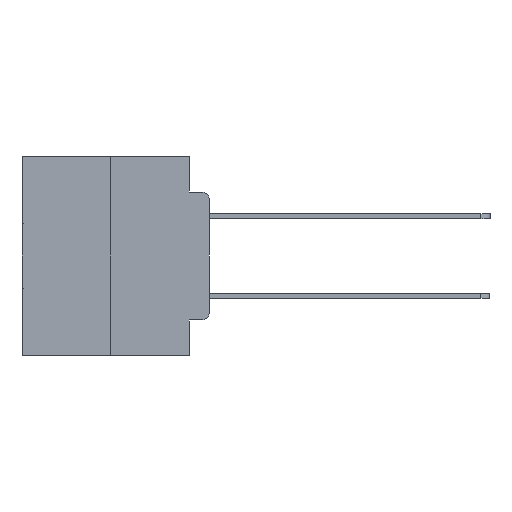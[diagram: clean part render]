
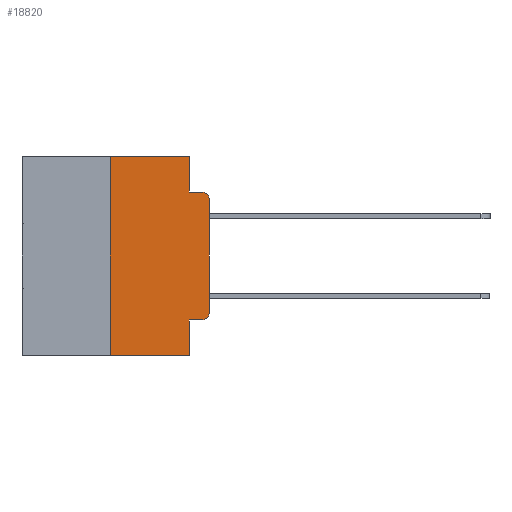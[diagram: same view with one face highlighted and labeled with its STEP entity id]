
A CAD part, left-side view. The second image highlights one B-rep face of the part: STEP entity #18820.
In plain terms, the highlighted planar face has unit normal (-1, 0, 0).
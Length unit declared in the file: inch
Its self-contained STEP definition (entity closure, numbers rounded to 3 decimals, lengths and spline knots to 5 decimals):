
#293 = DIRECTION ( 'NONE',  ( 0., 0., -1. ) ) ;
#661 = CARTESIAN_POINT ( 'NONE',  ( 0., 0., -0.1085 ) ) ;
#760 = VERTEX_POINT ( 'NONE', #27872 ) ;
#776 = ORIENTED_EDGE ( 'NONE', *, *, #23152, .F. ) ;
#808 = ORIENTED_EDGE ( 'NONE', *, *, #11839, .T. ) ;
#1389 = LINE ( 'NONE', #4992, #23170 ) ;
#1427 = CARTESIAN_POINT ( 'NONE',  ( 0., 0.473, 0. ) ) ;
#1507 = DIRECTION ( 'NONE',  ( 0., -1., 0. ) ) ;
#1617 = VERTEX_POINT ( 'NONE', #24075 ) ;
#1977 = LINE ( 'NONE', #11711, #16185 ) ;
#2202 = ORIENTED_EDGE ( 'NONE', *, *, #17604, .T. ) ;
#2776 = CARTESIAN_POINT ( 'NONE',  ( 0., 0.02, -0.3915 ) ) ;
#2945 = LINE ( 'NONE', #1427, #21610 ) ;
#3158 = VECTOR ( 'NONE', #23903, 39.37008 ) ;
#3261 = EDGE_CURVE ( 'NONE', #8089, #20990, #1389, .T. ) ;
#3321 = EDGE_CURVE ( 'NONE', #14280, #760, #9244, .T. ) ;
#3404 = VECTOR ( 'NONE', #19636, 39.37008 ) ;
#4658 = VECTOR ( 'NONE', #1507, 39.37008 ) ;
#4992 = CARTESIAN_POINT ( 'NONE',  ( 0., 0.25, 0. ) ) ;
#5052 = DIRECTION ( 'NONE',  ( 0., 0., -1. ) ) ;
#5710 = CARTESIAN_POINT ( 'NONE',  ( 0., 0.473, -0.5 ) ) ;
#6190 = VECTOR ( 'NONE', #25550, 39.37008 ) ;
#7208 = VERTEX_POINT ( 'NONE', #21252 ) ;
#7575 = DIRECTION ( 'NONE',  ( -1., 0., 0. ) ) ;
#7613 = VERTEX_POINT ( 'NONE', #661 ) ;
#7803 = DIRECTION ( 'NONE',  ( 0., 0., -1. ) ) ;
#8089 = VERTEX_POINT ( 'NONE', #12100 ) ;
#8682 = ORIENTED_EDGE ( 'NONE', *, *, #21087, .T. ) ;
#8787 = LINE ( 'NONE', #15295, #3404 ) ;
#9031 = ORIENTED_EDGE ( 'NONE', *, *, #3261, .F. ) ;
#9244 = LINE ( 'NONE', #18256, #3158 ) ;
#9692 = VERTEX_POINT ( 'NONE', #16600 ) ;
#10393 = EDGE_CURVE ( 'NONE', #7613, #760, #13295, .T. ) ;
#10438 = FACE_OUTER_BOUND ( 'NONE', #16031, .T. ) ;
#10463 = ORIENTED_EDGE ( 'NONE', *, *, #16174, .F. ) ;
#10605 = CARTESIAN_POINT ( 'NONE',  ( 0., 0.051, -0.5 ) ) ;
#10777 = LINE ( 'NONE', #12896, #4658 ) ;
#11406 = VECTOR ( 'NONE', #27967, 39.37008 ) ;
#11506 = ORIENTED_EDGE ( 'NONE', *, *, #3321, .F. ) ;
#11711 = CARTESIAN_POINT ( 'NONE',  ( 0., 0.051, 0. ) ) ;
#11839 = EDGE_CURVE ( 'NONE', #7208, #9692, #24347, .T. ) ;
#12100 = CARTESIAN_POINT ( 'NONE',  ( 0., 0.25, -0.5 ) ) ;
#12297 = LINE ( 'NONE', #18966, #6190 ) ;
#12302 = PLANE ( 'NONE',  #25947 ) ;
#12896 = CARTESIAN_POINT ( 'NONE',  ( 0., 0.051, -0.4115 ) ) ;
#13295 = CIRCLE ( 'NONE', #26937, 0.02 ) ;
#14280 = VERTEX_POINT ( 'NONE', #16419 ) ;
#15295 = CARTESIAN_POINT ( 'NONE',  ( 0., 0.051, 0. ) ) ;
#16031 = EDGE_LOOP ( 'NONE', ( #2202, #25005, #11506, #776, #26426, #9031, #8682, #10463, #18866, #808 ) ) ;
#16174 = EDGE_CURVE ( 'NONE', #1617, #16543, #1977, .T. ) ;
#16185 = VECTOR ( 'NONE', #293, 39.37008 ) ;
#16419 = CARTESIAN_POINT ( 'NONE',  ( 0., 0.051, -0.0885 ) ) ;
#16543 = VERTEX_POINT ( 'NONE', #10605 ) ;
#16600 = CARTESIAN_POINT ( 'NONE',  ( 0., 0., -0.3915 ) ) ;
#17285 = DIRECTION ( 'NONE',  ( 0., -1., 0. ) ) ;
#17604 = EDGE_CURVE ( 'NONE', #9692, #7613, #12297, .T. ) ;
#18256 = CARTESIAN_POINT ( 'NONE',  ( 0., 0.051, -0.0885 ) ) ;
#18400 = EDGE_CURVE ( 'NONE', #20990, #22371, #2945, .T. ) ;
#18599 = DIRECTION ( 'NONE',  ( -1., 0., 0. ) ) ;
#18820 = ADVANCED_FACE ( 'NONE', ( #10438 ), #12302, .F. ) ;
#18866 = ORIENTED_EDGE ( 'NONE', *, *, #19003, .T. ) ;
#18966 = CARTESIAN_POINT ( 'NONE',  ( 0., 0., 0. ) ) ;
#18998 = CARTESIAN_POINT ( 'NONE',  ( 0., 0.473, 0. ) ) ;
#19003 = EDGE_CURVE ( 'NONE', #1617, #7208, #10777, .T. ) ;
#19636 = DIRECTION ( 'NONE',  ( 0., 0., -1. ) ) ;
#19972 = AXIS2_PLACEMENT_3D ( 'NONE', #2776, #18599, #5052 ) ;
#20976 = CARTESIAN_POINT ( 'NONE',  ( 0., 0.25, 0. ) ) ;
#20990 = VERTEX_POINT ( 'NONE', #20976 ) ;
#21007 = CARTESIAN_POINT ( 'NONE',  ( 0., 0.02, -0.1085 ) ) ;
#21087 = EDGE_CURVE ( 'NONE', #8089, #16543, #27100, .T. ) ;
#21219 = DIRECTION ( 'NONE',  ( 1., 0., 0. ) ) ;
#21252 = CARTESIAN_POINT ( 'NONE',  ( 0., 0.02, -0.4115 ) ) ;
#21610 = VECTOR ( 'NONE', #17285, 39.37008 ) ;
#21815 = DIRECTION ( 'NONE',  ( 0., 0., 1. ) ) ;
#21941 = CARTESIAN_POINT ( 'NONE',  ( 0., 0.051, 0. ) ) ;
#22371 = VERTEX_POINT ( 'NONE', #21941 ) ;
#23152 = EDGE_CURVE ( 'NONE', #22371, #14280, #8787, .T. ) ;
#23170 = VECTOR ( 'NONE', #21815, 39.37008 ) ;
#23183 = DIRECTION ( 'NONE',  ( 0., 0., -1. ) ) ;
#23903 = DIRECTION ( 'NONE',  ( 0., -1., 0. ) ) ;
#24075 = CARTESIAN_POINT ( 'NONE',  ( 0., 0.051, -0.4115 ) ) ;
#24347 = CIRCLE ( 'NONE', #19972, 0.02 ) ;
#25005 = ORIENTED_EDGE ( 'NONE', *, *, #10393, .T. ) ;
#25550 = DIRECTION ( 'NONE',  ( 0., 0., 1. ) ) ;
#25947 = AXIS2_PLACEMENT_3D ( 'NONE', #18998, #21219, #7803 ) ;
#26426 = ORIENTED_EDGE ( 'NONE', *, *, #18400, .F. ) ;
#26937 = AXIS2_PLACEMENT_3D ( 'NONE', #21007, #7575, #23183 ) ;
#27100 = LINE ( 'NONE', #5710, #11406 ) ;
#27872 = CARTESIAN_POINT ( 'NONE',  ( 0., 0.02, -0.0885 ) ) ;
#27967 = DIRECTION ( 'NONE',  ( 0., -1., 0. ) ) ;
